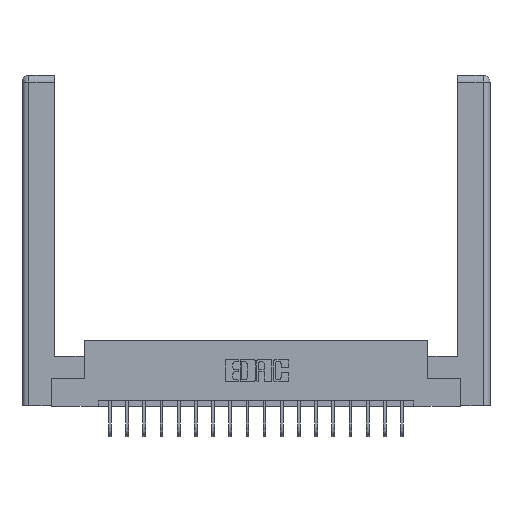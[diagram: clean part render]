
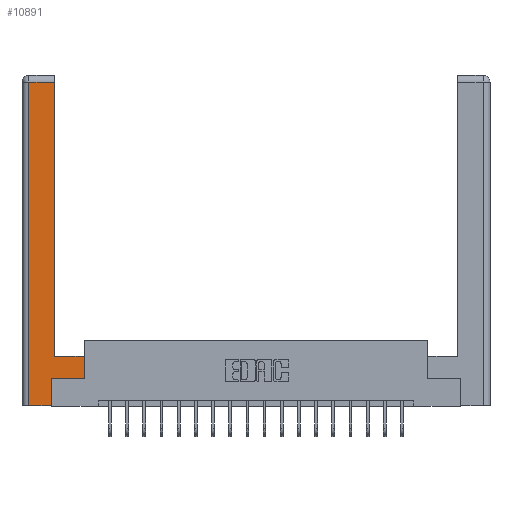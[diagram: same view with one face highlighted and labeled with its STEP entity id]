
A CAD part, top view. The second image highlights one B-rep face of the part: STEP entity #10891.
In plain terms, the highlighted planar face has unit normal (0, 0, 1).
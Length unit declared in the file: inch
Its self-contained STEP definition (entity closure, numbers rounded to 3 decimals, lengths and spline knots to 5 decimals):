
#80 = LINE ( 'NONE', #8921, #14246 ) ;
#328 = VECTOR ( 'NONE', #14289, 39.37008 ) ;
#439 = DIRECTION ( 'NONE',  ( 0., -1., 0. ) ) ;
#452 = DIRECTION ( 'NONE',  ( 1., 0., 0. ) ) ;
#1070 = CARTESIAN_POINT ( 'NONE',  ( 0.265, 0.245, 0. ) ) ;
#1100 = VERTEX_POINT ( 'NONE', #7272 ) ;
#1105 = LINE ( 'NONE', #13874, #4132 ) ;
#1245 = DIRECTION ( 'NONE',  ( -1., 0., 0. ) ) ;
#1389 = CARTESIAN_POINT ( 'NONE',  ( 0., 0., 0. ) ) ;
#1456 = CARTESIAN_POINT ( 'NONE',  ( 0.265, 0., 0. ) ) ;
#1592 = LINE ( 'NONE', #1070, #5079 ) ;
#2018 = VERTEX_POINT ( 'NONE', #11797 ) ;
#2173 = EDGE_CURVE ( 'NONE', #16676, #17113, #2604, .T. ) ;
#2479 = VERTEX_POINT ( 'NONE', #1456 ) ;
#2604 = LINE ( 'NONE', #10579, #3518 ) ;
#3091 = CARTESIAN_POINT ( 'NONE',  ( 0.0615, 2.94, 0. ) ) ;
#3238 = EDGE_CURVE ( 'NONE', #17113, #18727, #5169, .T. ) ;
#3518 = VECTOR ( 'NONE', #16716, 39.37008 ) ;
#4132 = VECTOR ( 'NONE', #452, 39.37008 ) ;
#4942 = ORIENTED_EDGE ( 'NONE', *, *, #13442, .T. ) ;
#5078 = EDGE_LOOP ( 'NONE', ( #13251, #4942, #5798, #9519, #11123, #12812, #13457, #7279 ) ) ;
#5079 = VECTOR ( 'NONE', #6954, 39.37008 ) ;
#5169 = LINE ( 'NONE', #17944, #18323 ) ;
#5595 = AXIS2_PLACEMENT_3D ( 'NONE', #1389, #8861, #1245 ) ;
#5798 = ORIENTED_EDGE ( 'NONE', *, *, #10900, .T. ) ;
#6283 = DIRECTION ( 'NONE',  ( -1., 0., 0. ) ) ;
#6925 = VECTOR ( 'NONE', #6283, 39.37008 ) ;
#6954 = DIRECTION ( 'NONE',  ( 0., 1., 0. ) ) ;
#7272 = CARTESIAN_POINT ( 'NONE',  ( 0.295, 2.94, 0. ) ) ;
#7279 = ORIENTED_EDGE ( 'NONE', *, *, #3238, .T. ) ;
#7673 = CARTESIAN_POINT ( 'NONE',  ( 0.0615, 2.94, 0. ) ) ;
#8861 = DIRECTION ( 'NONE',  ( 0., 0., -1. ) ) ;
#8921 = CARTESIAN_POINT ( 'NONE',  ( 0.0615, 0., 0. ) ) ;
#9519 = ORIENTED_EDGE ( 'NONE', *, *, #13960, .T. ) ;
#10130 = LINE ( 'NONE', #12801, #328 ) ;
#10579 = CARTESIAN_POINT ( 'NONE',  ( 0.565, 0.45, 0. ) ) ;
#10831 = CARTESIAN_POINT ( 'NONE',  ( 0.0615, 0., 0. ) ) ;
#10891 = ADVANCED_FACE ( 'NONE', ( #12180 ), #19120, .F. ) ;
#10900 = EDGE_CURVE ( 'NONE', #19006, #17397, #80, .T. ) ;
#11123 = ORIENTED_EDGE ( 'NONE', *, *, #12449, .T. ) ;
#11797 = CARTESIAN_POINT ( 'NONE',  ( 0.265, 0.245, 0. ) ) ;
#12025 = CARTESIAN_POINT ( 'NONE',  ( 0.295, 3., 0. ) ) ;
#12047 = CARTESIAN_POINT ( 'NONE',  ( 0.565, 0.245, 0. ) ) ;
#12180 = FACE_OUTER_BOUND ( 'NONE', #5078, .T. ) ;
#12449 = EDGE_CURVE ( 'NONE', #2479, #2018, #1592, .T. ) ;
#12547 = EDGE_CURVE ( 'NONE', #18727, #1100, #17374, .T. ) ;
#12801 = CARTESIAN_POINT ( 'NONE',  ( 0.265, 0., 0. ) ) ;
#12812 = ORIENTED_EDGE ( 'NONE', *, *, #19047, .T. ) ;
#13251 = ORIENTED_EDGE ( 'NONE', *, *, #12547, .T. ) ;
#13442 = EDGE_CURVE ( 'NONE', #1100, #19006, #17334, .T. ) ;
#13457 = ORIENTED_EDGE ( 'NONE', *, *, #2173, .T. ) ;
#13874 = CARTESIAN_POINT ( 'NONE',  ( 0.565, 0.245, 0. ) ) ;
#13960 = EDGE_CURVE ( 'NONE', #17397, #2479, #10130, .T. ) ;
#14134 = CARTESIAN_POINT ( 'NONE',  ( 0.565, 0.45, 0. ) ) ;
#14246 = VECTOR ( 'NONE', #439, 39.37008 ) ;
#14289 = DIRECTION ( 'NONE',  ( 1., 0., 0. ) ) ;
#15032 = DIRECTION ( 'NONE',  ( -1., 0., 0. ) ) ;
#15580 = CARTESIAN_POINT ( 'NONE',  ( 0.295, 0.45, 0. ) ) ;
#16253 = DIRECTION ( 'NONE',  ( 0., 1., 0. ) ) ;
#16676 = VERTEX_POINT ( 'NONE', #12047 ) ;
#16716 = DIRECTION ( 'NONE',  ( 0., 1., 0. ) ) ;
#17113 = VERTEX_POINT ( 'NONE', #14134 ) ;
#17334 = LINE ( 'NONE', #3091, #6925 ) ;
#17374 = LINE ( 'NONE', #12025, #18262 ) ;
#17397 = VERTEX_POINT ( 'NONE', #10831 ) ;
#17944 = CARTESIAN_POINT ( 'NONE',  ( 0.295, 0.45, 0. ) ) ;
#18262 = VECTOR ( 'NONE', #16253, 39.37008 ) ;
#18323 = VECTOR ( 'NONE', #15032, 39.37008 ) ;
#18727 = VERTEX_POINT ( 'NONE', #15580 ) ;
#19006 = VERTEX_POINT ( 'NONE', #7673 ) ;
#19047 = EDGE_CURVE ( 'NONE', #2018, #16676, #1105, .T. ) ;
#19120 = PLANE ( 'NONE',  #5595 ) ;
